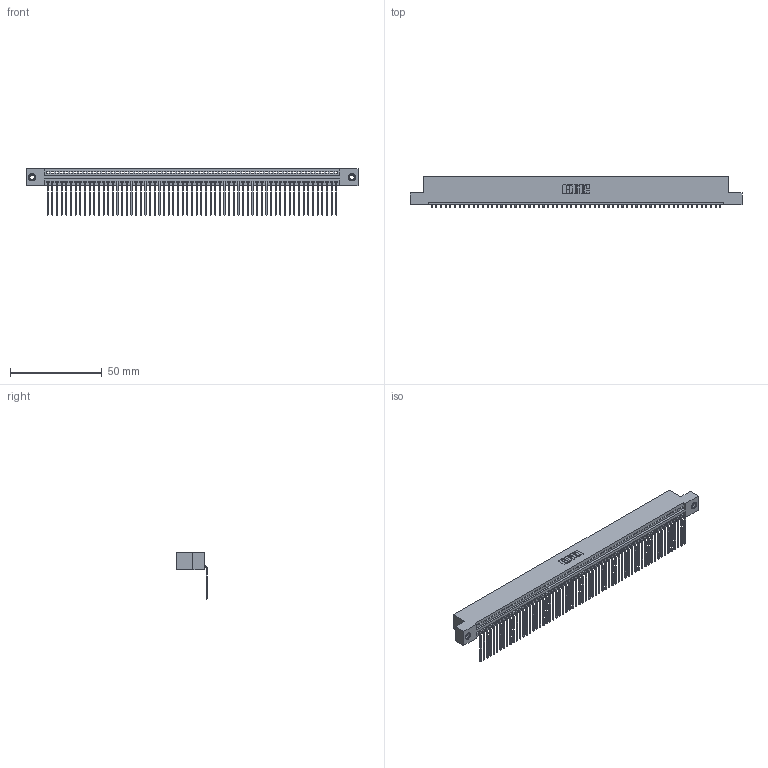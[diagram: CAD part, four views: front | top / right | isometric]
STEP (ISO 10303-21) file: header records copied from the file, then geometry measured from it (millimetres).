
FILE_DESCRIPTION (( 'STEP AP203' ), '1' );
FILE_NAME ('395-063-559-107.STEP', '2018-11-24T10:51:47', ( '' ), ( '' ), 'SwSTEP 2.0', 'SolidWorks 2016', '' );
FILE_SCHEMA (( 'CONFIG_CONTROL_DESIGN' ));
Length unit declared in the file: inch
Products named in the file (4): 345-292-001_558 559 Tail - 1; 395-063-559-107; 345 Part_Flush Mounting Lugs - 0.156 Dia-TI; 345-250-001_345-250-005-103
Assembly tree (66 placements, depth 2):
  395-063-559-107
    345 Part_Flush Mounting Lugs - 0.156 Dia-TI
    345-292-001_558 559 Tail - 1  x63
    345-250-001_345-250-005-103  x2
Bounding box: 181.23 x 16.75 x 25.53 mm (x, y, z)
Volume: 17581.7 mm3; surface area: 24915.9 mm2
Topology: 66 solids, 66 shells, 3966 faces, 11943 edges, 7870 vertices
Faces by surface type: plane 2758, cylinder 1192, cone 12, torus 4
Entity records: 45858 total; most frequent: CARTESIAN_POINT 7924, ORIENTED_EDGE 7914, DIRECTION 6917, EDGE_CURVE 3957, VECTOR 3553, LINE 3553, VERTEX_POINT 2632, AXIS2_PLACEMENT_3D 1682
